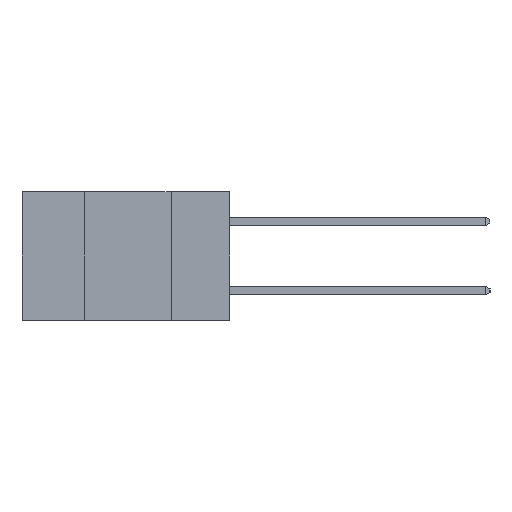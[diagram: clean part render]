
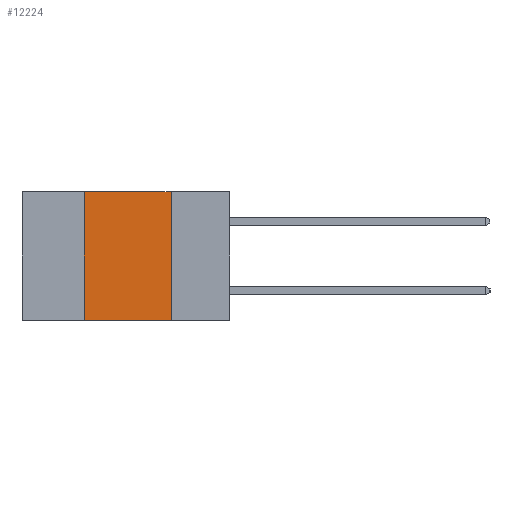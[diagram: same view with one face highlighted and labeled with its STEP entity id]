
A CAD part, left-side view. The second image highlights one B-rep face of the part: STEP entity #12224.
In plain terms, the highlighted planar face has unit normal (-1, 0, 0).
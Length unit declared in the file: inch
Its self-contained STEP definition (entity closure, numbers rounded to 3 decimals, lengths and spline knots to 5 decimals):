
#124 = CARTESIAN_POINT ( 'NONE',  ( 0., 0.6, -0.37 ) ) ;
#348 = CARTESIAN_POINT ( 'NONE',  ( 0., 0.42, 0. ) ) ;
#853 = ORIENTED_EDGE ( 'NONE', *, *, #10356, .F. ) ;
#897 = FACE_OUTER_BOUND ( 'NONE', #2636, .T. ) ;
#1793 = LINE ( 'NONE', #6461, #12995 ) ;
#1795 = CARTESIAN_POINT ( 'NONE',  ( 0., 0.6, 0. ) ) ;
#1986 = EDGE_CURVE ( 'NONE', #3726, #7796, #8341, .T. ) ;
#2636 = EDGE_LOOP ( 'NONE', ( #12781, #853, #9366, #7804 ) ) ;
#2844 = VECTOR ( 'NONE', #6209, 39.37008 ) ;
#3204 = LINE ( 'NONE', #1795, #2844 ) ;
#3420 = AXIS2_PLACEMENT_3D ( 'NONE', #7256, #12637, #6166 ) ;
#3726 = VERTEX_POINT ( 'NONE', #10522 ) ;
#5051 = PLANE ( 'NONE',  #3420 ) ;
#5781 = CARTESIAN_POINT ( 'NONE',  ( 0., 0.17, 0. ) ) ;
#5870 = CARTESIAN_POINT ( 'NONE',  ( 0., 0.42, -0.37 ) ) ;
#5917 = EDGE_CURVE ( 'NONE', #6007, #7796, #1793, .T. ) ;
#6007 = VERTEX_POINT ( 'NONE', #5781 ) ;
#6046 = LINE ( 'NONE', #5870, #11526 ) ;
#6166 = DIRECTION ( 'NONE',  ( 0., 0., -1. ) ) ;
#6209 = DIRECTION ( 'NONE',  ( 0., -1., 0. ) ) ;
#6358 = DIRECTION ( 'NONE',  ( 0., 0., -1. ) ) ;
#6461 = CARTESIAN_POINT ( 'NONE',  ( 0., 0.17, -0.37 ) ) ;
#7016 = DIRECTION ( 'NONE',  ( 0., 0., 1. ) ) ;
#7256 = CARTESIAN_POINT ( 'NONE',  ( 0., 0.6, 0. ) ) ;
#7796 = VERTEX_POINT ( 'NONE', #12311 ) ;
#7804 = ORIENTED_EDGE ( 'NONE', *, *, #1986, .T. ) ;
#7983 = VECTOR ( 'NONE', #13819, 39.37008 ) ;
#8341 = LINE ( 'NONE', #124, #7983 ) ;
#9366 = ORIENTED_EDGE ( 'NONE', *, *, #13150, .F. ) ;
#10356 = EDGE_CURVE ( 'NONE', #13130, #6007, #3204, .T. ) ;
#10522 = CARTESIAN_POINT ( 'NONE',  ( 0., 0.42, -0.37 ) ) ;
#11526 = VECTOR ( 'NONE', #7016, 39.37008 ) ;
#12224 = ADVANCED_FACE ( 'NONE', ( #897 ), #5051, .F. ) ;
#12311 = CARTESIAN_POINT ( 'NONE',  ( 0., 0.17, -0.37 ) ) ;
#12637 = DIRECTION ( 'NONE',  ( 1., 0., 0. ) ) ;
#12781 = ORIENTED_EDGE ( 'NONE', *, *, #5917, .F. ) ;
#12995 = VECTOR ( 'NONE', #6358, 39.37008 ) ;
#13130 = VERTEX_POINT ( 'NONE', #348 ) ;
#13150 = EDGE_CURVE ( 'NONE', #3726, #13130, #6046, .T. ) ;
#13819 = DIRECTION ( 'NONE',  ( 0., -1., 0. ) ) ;
